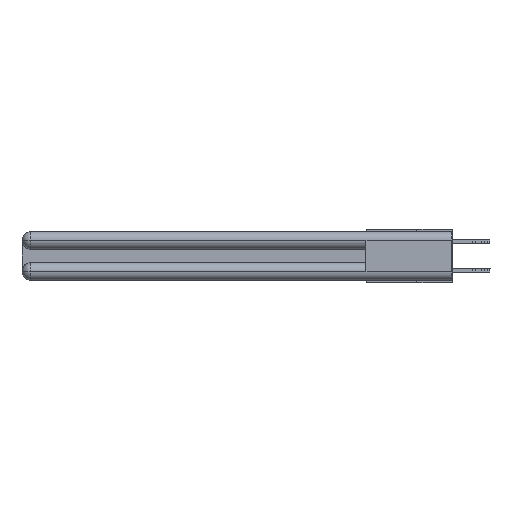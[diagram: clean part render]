
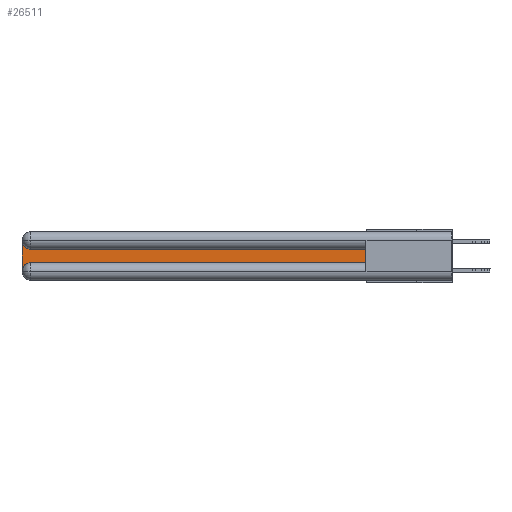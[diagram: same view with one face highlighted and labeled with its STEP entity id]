
A CAD part, left-side view. The second image highlights one B-rep face of the part: STEP entity #26511.
In plain terms, the highlighted planar face has unit normal (-1, 0, 0).
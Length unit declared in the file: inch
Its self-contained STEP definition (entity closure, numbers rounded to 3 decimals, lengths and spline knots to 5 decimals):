
#77 = DIRECTION ( 'NONE',  ( 0., 0., 1. ) ) ;
#1308 = PLANE ( 'NONE',  #8327 ) ;
#1842 = ORIENTED_EDGE ( 'NONE', *, *, #7057, .T. ) ;
#2115 = ORIENTED_EDGE ( 'NONE', *, *, #28022, .T. ) ;
#2287 = CARTESIAN_POINT ( 'NONE',  ( 0.075, 0.6, -0.2175 ) ) ;
#2801 = CARTESIAN_POINT ( 'NONE',  ( 0.075, 0.6, -0.1225 ) ) ;
#4516 = CARTESIAN_POINT ( 'NONE',  ( 0.075, 0.6, -0.2175 ) ) ;
#5298 = DIRECTION ( 'NONE',  ( 0., 0., -1. ) ) ;
#5535 = VERTEX_POINT ( 'NONE', #17018 ) ;
#5599 = VERTEX_POINT ( 'NONE', #7861 ) ;
#7057 = EDGE_CURVE ( 'NONE', #23646, #5599, #26940, .T. ) ;
#7370 = LINE ( 'NONE', #22694, #9790 ) ;
#7701 = EDGE_LOOP ( 'NONE', ( #24867, #23327, #2115, #1842, #8301, #19930 ) ) ;
#7861 = CARTESIAN_POINT ( 'NONE',  ( 0.075, 2.94, -0.2175 ) ) ;
#8301 = ORIENTED_EDGE ( 'NONE', *, *, #12908, .T. ) ;
#8327 = AXIS2_PLACEMENT_3D ( 'NONE', #28027, #12289, #27749 ) ;
#8673 = VECTOR ( 'NONE', #24263, 39.37008 ) ;
#9003 = FACE_OUTER_BOUND ( 'NONE', #7701, .T. ) ;
#9604 = LINE ( 'NONE', #13381, #25467 ) ;
#9790 = VECTOR ( 'NONE', #22406, 39.37008 ) ;
#10210 = VERTEX_POINT ( 'NONE', #2801 ) ;
#10801 = EDGE_CURVE ( 'NONE', #10210, #5535, #7370, .T. ) ;
#11328 = VERTEX_POINT ( 'NONE', #22791 ) ;
#12289 = DIRECTION ( 'NONE',  ( 1., 0., 0. ) ) ;
#12908 = EDGE_CURVE ( 'NONE', #5599, #16642, #13872, .T. ) ;
#13119 = CARTESIAN_POINT ( 'NONE',  ( 0.075, 2.94, -0.2775 ) ) ;
#13381 = CARTESIAN_POINT ( 'NONE',  ( 0.075, 0.6, -0.2175 ) ) ;
#13872 = LINE ( 'NONE', #2287, #8673 ) ;
#14294 = EDGE_CURVE ( 'NONE', #16642, #10210, #9604, .T. ) ;
#14705 = CARTESIAN_POINT ( 'NONE',  ( 0.075, 3., -0.2775 ) ) ;
#15431 = VECTOR ( 'NONE', #5298, 39.37008 ) ;
#16156 = CARTESIAN_POINT ( 'NONE',  ( 0.075, 2.94, -0.0625 ) ) ;
#16489 = LINE ( 'NONE', #18543, #15431 ) ;
#16642 = VERTEX_POINT ( 'NONE', #4516 ) ;
#17018 = CARTESIAN_POINT ( 'NONE',  ( 0.075, 2.94, -0.1225 ) ) ;
#18009 = DIRECTION ( 'NONE',  ( 1., 0., 0. ) ) ;
#18543 = CARTESIAN_POINT ( 'NONE',  ( 0.075, 3., -0.2175 ) ) ;
#19669 = CIRCLE ( 'NONE', #27017, 0.06 ) ;
#19750 = DIRECTION ( 'NONE',  ( 0., 0., -1. ) ) ;
#19930 = ORIENTED_EDGE ( 'NONE', *, *, #14294, .T. ) ;
#22406 = DIRECTION ( 'NONE',  ( 0., 1., 0. ) ) ;
#22463 = DIRECTION ( 'NONE',  ( 0., 0., -1. ) ) ;
#22694 = CARTESIAN_POINT ( 'NONE',  ( 0.075, 0.6, -0.1225 ) ) ;
#22791 = CARTESIAN_POINT ( 'NONE',  ( 0.075, 3., -0.0625 ) ) ;
#23327 = ORIENTED_EDGE ( 'NONE', *, *, #27099, .T. ) ;
#23646 = VERTEX_POINT ( 'NONE', #14705 ) ;
#24263 = DIRECTION ( 'NONE',  ( 0., -1., 0. ) ) ;
#24867 = ORIENTED_EDGE ( 'NONE', *, *, #10801, .T. ) ;
#25467 = VECTOR ( 'NONE', #77, 39.37008 ) ;
#26511 = ADVANCED_FACE ( 'NONE', ( #9003 ), #1308, .F. ) ;
#26940 = CIRCLE ( 'NONE', #27337, 0.06 ) ;
#27017 = AXIS2_PLACEMENT_3D ( 'NONE', #16156, #18009, #22463 ) ;
#27099 = EDGE_CURVE ( 'NONE', #5535, #11328, #19669, .T. ) ;
#27337 = AXIS2_PLACEMENT_3D ( 'NONE', #13119, #28379, #19750 ) ;
#27749 = DIRECTION ( 'NONE',  ( 0., 0., -1. ) ) ;
#28022 = EDGE_CURVE ( 'NONE', #11328, #23646, #16489, .T. ) ;
#28027 = CARTESIAN_POINT ( 'NONE',  ( 0.075, 3., -0.1225 ) ) ;
#28379 = DIRECTION ( 'NONE',  ( 1., 0., 0. ) ) ;
